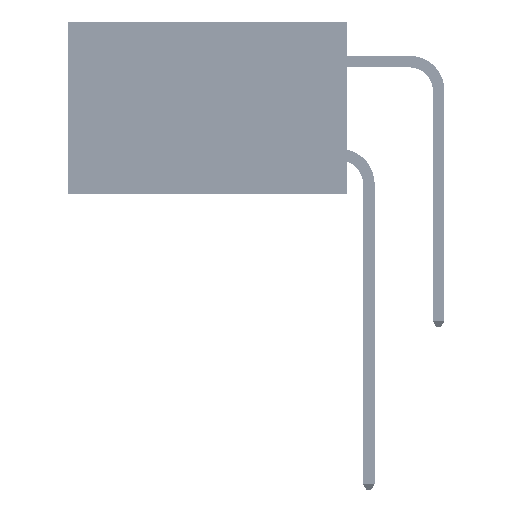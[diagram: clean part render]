
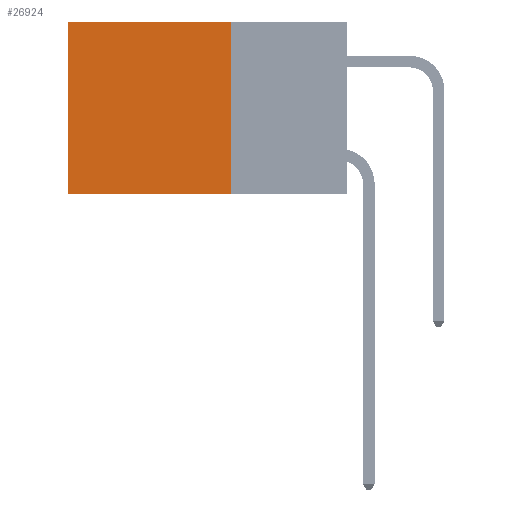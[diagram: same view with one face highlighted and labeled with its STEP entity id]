
A CAD part, left-side view. The second image highlights one B-rep face of the part: STEP entity #26924.
In plain terms, the highlighted planar face has unit normal (-1, 0, 0).
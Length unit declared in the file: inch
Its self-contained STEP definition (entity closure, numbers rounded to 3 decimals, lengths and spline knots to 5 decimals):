
#592 = EDGE_CURVE ( 'NONE', #6310, #28609, #40951, .T. ) ;
#1101 = VECTOR ( 'NONE', #21734, 39.37008 ) ;
#2591 = EDGE_CURVE ( 'NONE', #6310, #40071, #24498, .T. ) ;
#2801 = PLANE ( 'NONE',  #32672 ) ;
#5576 = CARTESIAN_POINT ( 'NONE',  ( 0.2875, 0.6, 0. ) ) ;
#6310 = VERTEX_POINT ( 'NONE', #9633 ) ;
#6408 = VERTEX_POINT ( 'NONE', #13923 ) ;
#9633 = CARTESIAN_POINT ( 'NONE',  ( 0.2875, 0.25, 0. ) ) ;
#10219 = ORIENTED_EDGE ( 'NONE', *, *, #43536, .F. ) ;
#10776 = DIRECTION ( 'NONE',  ( 1., 0., 0. ) ) ;
#10847 = CARTESIAN_POINT ( 'NONE',  ( 0.2875, 0.25, 0. ) ) ;
#11667 = LINE ( 'NONE', #44811, #1101 ) ;
#13026 = CARTESIAN_POINT ( 'NONE',  ( 0.2875, 0.25, -0.37 ) ) ;
#13715 = EDGE_LOOP ( 'NONE', ( #32383, #10219, #48867, #35887 ) ) ;
#13923 = CARTESIAN_POINT ( 'NONE',  ( 0.2875, 0.6, -0.37 ) ) ;
#14599 = DIRECTION ( 'NONE',  ( 0., 0., -1. ) ) ;
#16003 = LINE ( 'NONE', #13026, #45547 ) ;
#18013 = VECTOR ( 'NONE', #33513, 39.37008 ) ;
#20315 = EDGE_CURVE ( 'NONE', #28609, #6408, #11667, .T. ) ;
#21087 = CARTESIAN_POINT ( 'NONE',  ( 0.2875, 0.25, -0.37 ) ) ;
#21734 = DIRECTION ( 'NONE',  ( 0., 0., -1. ) ) ;
#24498 = LINE ( 'NONE', #10847, #43776 ) ;
#26924 = ADVANCED_FACE ( 'NONE', ( #43615 ), #2801, .F. ) ;
#28609 = VERTEX_POINT ( 'NONE', #5576 ) ;
#29618 = CARTESIAN_POINT ( 'NONE',  ( 0.2875, 0.25, 0. ) ) ;
#32383 = ORIENTED_EDGE ( 'NONE', *, *, #20315, .T. ) ;
#32672 = AXIS2_PLACEMENT_3D ( 'NONE', #33965, #10776, #37829 ) ;
#33513 = DIRECTION ( 'NONE',  ( 0., 1., 0. ) ) ;
#33965 = CARTESIAN_POINT ( 'NONE',  ( 0.2875, 0.25, 0. ) ) ;
#35887 = ORIENTED_EDGE ( 'NONE', *, *, #592, .T. ) ;
#36182 = DIRECTION ( 'NONE',  ( 0., 1., 0. ) ) ;
#37829 = DIRECTION ( 'NONE',  ( 0., 0., -1. ) ) ;
#40071 = VERTEX_POINT ( 'NONE', #21087 ) ;
#40951 = LINE ( 'NONE', #29618, #18013 ) ;
#43536 = EDGE_CURVE ( 'NONE', #40071, #6408, #16003, .T. ) ;
#43615 = FACE_OUTER_BOUND ( 'NONE', #13715, .T. ) ;
#43776 = VECTOR ( 'NONE', #14599, 39.37008 ) ;
#44811 = CARTESIAN_POINT ( 'NONE',  ( 0.2875, 0.6, 0. ) ) ;
#45547 = VECTOR ( 'NONE', #36182, 39.37008 ) ;
#48867 = ORIENTED_EDGE ( 'NONE', *, *, #2591, .F. ) ;
